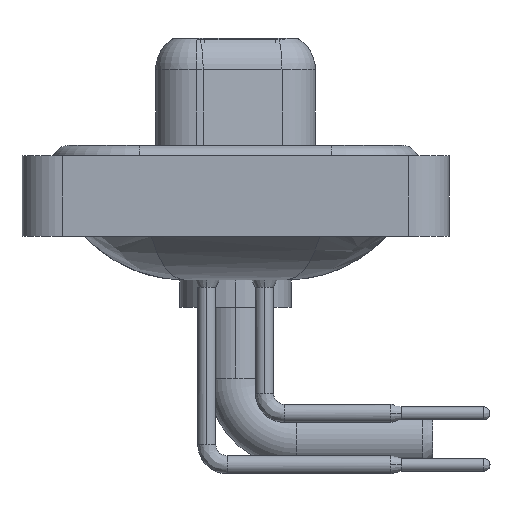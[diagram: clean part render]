
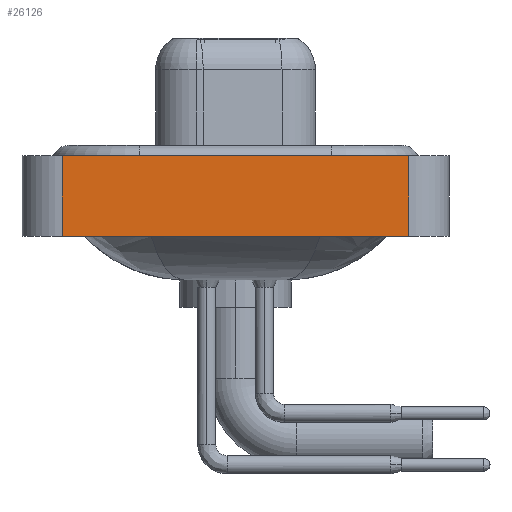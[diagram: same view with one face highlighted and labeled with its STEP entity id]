
A CAD part, left-side view. The second image highlights one B-rep face of the part: STEP entity #26126.
In plain terms, the highlighted planar face has unit normal (-1, 0, 0).
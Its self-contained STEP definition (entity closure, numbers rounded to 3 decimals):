
#421 = CARTESIAN_POINT ( 'NONE',  ( -7.35, -8.55, 0.4 ) ) ;
#452 = EDGE_CURVE ( 'NONE', #2718, #15332, #21866, .T. ) ;
#2718 = VERTEX_POINT ( 'NONE', #15914 ) ;
#3648 = DIRECTION ( 'NONE',  ( 0., 0., 1. ) ) ;
#3854 = LINE ( 'NONE', #19708, #16201 ) ;
#3860 = ORIENTED_EDGE ( 'NONE', *, *, #5282, .F. ) ;
#5282 = EDGE_CURVE ( 'NONE', #18179, #15332, #10085, .T. ) ;
#6511 = DIRECTION ( 'NONE',  ( 0., 0., 1. ) ) ;
#7750 = AXIS2_PLACEMENT_3D ( 'NONE', #18349, #10256, #6511 ) ;
#8774 = ORIENTED_EDGE ( 'NONE', *, *, #8949, .T. ) ;
#8949 = EDGE_CURVE ( 'NONE', #11881, #2718, #12303, .T. ) ;
#10085 = LINE ( 'NONE', #18169, #16242 ) ;
#10256 = DIRECTION ( 'NONE',  ( -1., 0., 0. ) ) ;
#10301 = CARTESIAN_POINT ( 'NONE',  ( -7.35, -8.55, -3.6 ) ) ;
#11881 = VERTEX_POINT ( 'NONE', #22477 ) ;
#12303 = LINE ( 'NONE', #10301, #15950 ) ;
#14015 = DIRECTION ( 'NONE',  ( 0., 0., 1. ) ) ;
#14394 = FACE_OUTER_BOUND ( 'NONE', #16272, .T. ) ;
#15332 = VERTEX_POINT ( 'NONE', #421 ) ;
#15914 = CARTESIAN_POINT ( 'NONE',  ( -7.35, -8.55, -3.6 ) ) ;
#15950 = VECTOR ( 'NONE', #18395, 1000. ) ;
#16201 = VECTOR ( 'NONE', #14015, 1000. ) ;
#16242 = VECTOR ( 'NONE', #23885, 1000. ) ;
#16272 = EDGE_LOOP ( 'NONE', ( #21232, #3860, #19003, #8774 ) ) ;
#16637 = PLANE ( 'NONE',  #7750 ) ;
#18015 = CARTESIAN_POINT ( 'NONE',  ( -7.35, -8.55, -3.6 ) ) ;
#18169 = CARTESIAN_POINT ( 'NONE',  ( -7.35, -8.55, 0.4 ) ) ;
#18179 = VERTEX_POINT ( 'NONE', #23983 ) ;
#18349 = CARTESIAN_POINT ( 'NONE',  ( -7.35, -8.55, -3.6 ) ) ;
#18395 = DIRECTION ( 'NONE',  ( 0., -1., 0. ) ) ;
#19003 = ORIENTED_EDGE ( 'NONE', *, *, #23602, .F. ) ;
#19708 = CARTESIAN_POINT ( 'NONE',  ( -7.35, 8.55, -3.6 ) ) ;
#21232 = ORIENTED_EDGE ( 'NONE', *, *, #452, .T. ) ;
#21866 = LINE ( 'NONE', #18015, #23227 ) ;
#22477 = CARTESIAN_POINT ( 'NONE',  ( -7.35, 8.55, -3.6 ) ) ;
#23227 = VECTOR ( 'NONE', #3648, 1000. ) ;
#23602 = EDGE_CURVE ( 'NONE', #11881, #18179, #3854, .T. ) ;
#23885 = DIRECTION ( 'NONE',  ( 0., -1., 0. ) ) ;
#23983 = CARTESIAN_POINT ( 'NONE',  ( -7.35, 8.55, 0.4 ) ) ;
#26126 = ADVANCED_FACE ( 'NONE', ( #14394 ), #16637, .T. ) ;
